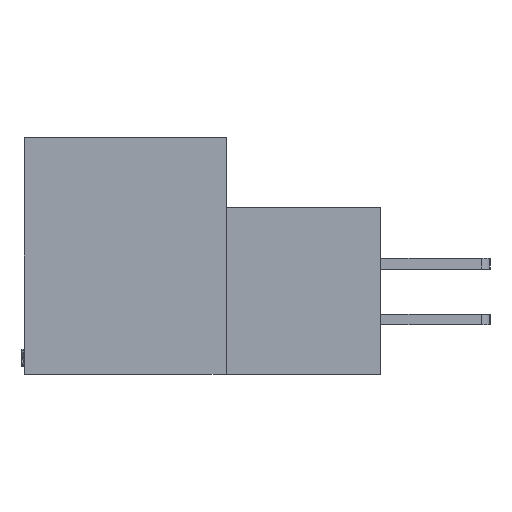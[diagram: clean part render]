
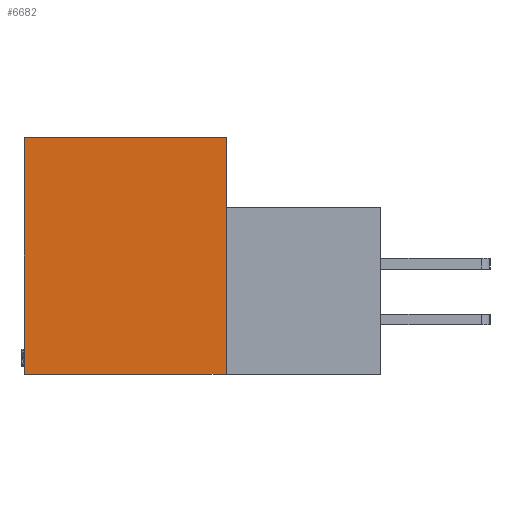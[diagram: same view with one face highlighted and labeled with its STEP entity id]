
A CAD part, left-side view. The second image highlights one B-rep face of the part: STEP entity #6682.
In plain terms, the highlighted planar face has unit normal (-1, 0, 0).
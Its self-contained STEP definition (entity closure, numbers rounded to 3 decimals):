
#597 = PLANE ( 'NONE',  #12190 ) ;
#1915 = VECTOR ( 'NONE', #27564, 1000. ) ;
#1929 = CARTESIAN_POINT ( 'NONE',  ( 0., 0., -13.487 ) ) ;
#4033 = VERTEX_POINT ( 'NONE', #18524 ) ;
#4160 = LINE ( 'NONE', #29256, #16954 ) ;
#4641 = CARTESIAN_POINT ( 'NONE',  ( 0., 11.506, 0. ) ) ;
#5840 = EDGE_LOOP ( 'NONE', ( #20235, #16001, #6858, #13659 ) ) ;
#6682 = ADVANCED_FACE ( 'NONE', ( #7579 ), #597, .F. ) ;
#6717 = EDGE_CURVE ( 'NONE', #4033, #14138, #28595, .T. ) ;
#6858 = ORIENTED_EDGE ( 'NONE', *, *, #19228, .F. ) ;
#7083 = EDGE_CURVE ( 'NONE', #10628, #20005, #15740, .T. ) ;
#7536 = CARTESIAN_POINT ( 'NONE',  ( 0., 0., 0. ) ) ;
#7579 = FACE_OUTER_BOUND ( 'NONE', #5840, .T. ) ;
#8455 = DIRECTION ( 'NONE',  ( 0., -1., 0. ) ) ;
#9742 = DIRECTION ( 'NONE',  ( 0., 0., -1. ) ) ;
#10628 = VERTEX_POINT ( 'NONE', #11148 ) ;
#11148 = CARTESIAN_POINT ( 'NONE',  ( 0., 11.506, -13.487 ) ) ;
#12158 = LINE ( 'NONE', #13051, #28181 ) ;
#12190 = AXIS2_PLACEMENT_3D ( 'NONE', #25258, #16605, #9742 ) ;
#12551 = VECTOR ( 'NONE', #13500, 1000. ) ;
#13051 = CARTESIAN_POINT ( 'NONE',  ( 0., 11.506, 0. ) ) ;
#13247 = DIRECTION ( 'NONE',  ( 0., 1., 0. ) ) ;
#13500 = DIRECTION ( 'NONE',  ( 0., 0., 1. ) ) ;
#13659 = ORIENTED_EDGE ( 'NONE', *, *, #7083, .F. ) ;
#14138 = VERTEX_POINT ( 'NONE', #1929 ) ;
#14146 = EDGE_CURVE ( 'NONE', #14138, #10628, #4160, .T. ) ;
#15740 = LINE ( 'NONE', #24647, #12551 ) ;
#16001 = ORIENTED_EDGE ( 'NONE', *, *, #6717, .F. ) ;
#16605 = DIRECTION ( 'NONE',  ( 1., 0., 0. ) ) ;
#16954 = VECTOR ( 'NONE', #13247, 1000. ) ;
#18524 = CARTESIAN_POINT ( 'NONE',  ( 0., 0., 0. ) ) ;
#19228 = EDGE_CURVE ( 'NONE', #20005, #4033, #12158, .T. ) ;
#20005 = VERTEX_POINT ( 'NONE', #4641 ) ;
#20235 = ORIENTED_EDGE ( 'NONE', *, *, #14146, .F. ) ;
#24647 = CARTESIAN_POINT ( 'NONE',  ( 0., 11.506, -13.487 ) ) ;
#25258 = CARTESIAN_POINT ( 'NONE',  ( 0., 0., 0. ) ) ;
#27564 = DIRECTION ( 'NONE',  ( 0., 0., -1. ) ) ;
#28181 = VECTOR ( 'NONE', #8455, 1000. ) ;
#28595 = LINE ( 'NONE', #7536, #1915 ) ;
#29256 = CARTESIAN_POINT ( 'NONE',  ( 0., -8.814, -13.487 ) ) ;
